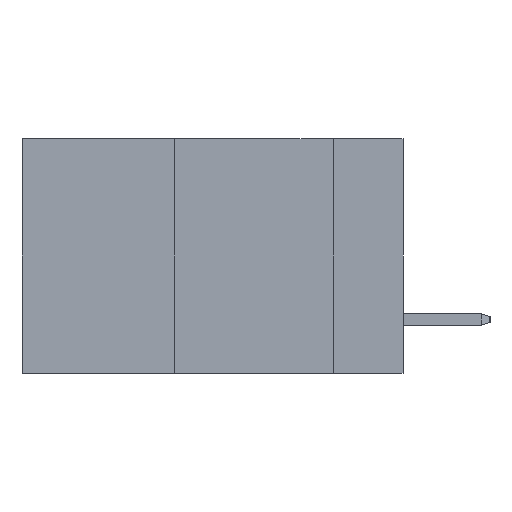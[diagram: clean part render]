
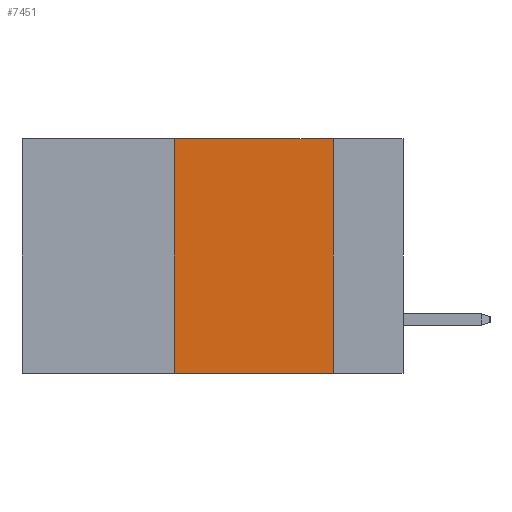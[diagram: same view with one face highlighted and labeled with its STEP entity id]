
A CAD part, left-side view. The second image highlights one B-rep face of the part: STEP entity #7451.
In plain terms, the highlighted planar face has unit normal (-1, 0, 0).
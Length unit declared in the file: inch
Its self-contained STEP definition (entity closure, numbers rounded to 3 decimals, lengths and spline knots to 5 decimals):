
#170 = DIRECTION ( 'NONE',  ( 0., -1., 0. ) ) ;
#464 = EDGE_CURVE ( 'NONE', #6376, #3207, #1297, .T. ) ;
#1163 = DIRECTION ( 'NONE',  ( 1., 0., 0. ) ) ;
#1297 = LINE ( 'NONE', #16096, #6875 ) ;
#2264 = CARTESIAN_POINT ( 'NONE',  ( 0., 0.36, 0. ) ) ;
#2473 = CARTESIAN_POINT ( 'NONE',  ( 0., 0.36, 0. ) ) ;
#2484 = PLANE ( 'NONE',  #2723 ) ;
#2723 = AXIS2_PLACEMENT_3D ( 'NONE', #7893, #1163, #16060 ) ;
#3059 = LINE ( 'NONE', #8479, #6296 ) ;
#3207 = VERTEX_POINT ( 'NONE', #8683 ) ;
#3241 = LINE ( 'NONE', #16770, #14973 ) ;
#3449 = ORIENTED_EDGE ( 'NONE', *, *, #464, .F. ) ;
#3927 = CARTESIAN_POINT ( 'NONE',  ( 0., 0.11, 0. ) ) ;
#6296 = VECTOR ( 'NONE', #12302, 39.37008 ) ;
#6376 = VERTEX_POINT ( 'NONE', #3927 ) ;
#6842 = CARTESIAN_POINT ( 'NONE',  ( 0., 0.36, -0.37 ) ) ;
#6875 = VECTOR ( 'NONE', #17376, 39.37008 ) ;
#7451 = ADVANCED_FACE ( 'NONE', ( #14648 ), #2484, .F. ) ;
#7579 = LINE ( 'NONE', #2264, #11008 ) ;
#7796 = ORIENTED_EDGE ( 'NONE', *, *, #17082, .F. ) ;
#7893 = CARTESIAN_POINT ( 'NONE',  ( 0., 0.6, 0. ) ) ;
#8479 = CARTESIAN_POINT ( 'NONE',  ( 0., 0.6, 0. ) ) ;
#8683 = CARTESIAN_POINT ( 'NONE',  ( 0., 0.11, -0.37 ) ) ;
#9094 = ORIENTED_EDGE ( 'NONE', *, *, #9726, .T. ) ;
#9726 = EDGE_CURVE ( 'NONE', #10562, #3207, #3241, .T. ) ;
#9874 = EDGE_CURVE ( 'NONE', #10562, #12164, #7579, .T. ) ;
#10342 = DIRECTION ( 'NONE',  ( 0., 0., 1. ) ) ;
#10562 = VERTEX_POINT ( 'NONE', #6842 ) ;
#11008 = VECTOR ( 'NONE', #10342, 39.37008 ) ;
#12164 = VERTEX_POINT ( 'NONE', #2473 ) ;
#12302 = DIRECTION ( 'NONE',  ( 0., -1., 0. ) ) ;
#12348 = ORIENTED_EDGE ( 'NONE', *, *, #9874, .F. ) ;
#14312 = EDGE_LOOP ( 'NONE', ( #3449, #7796, #12348, #9094 ) ) ;
#14648 = FACE_OUTER_BOUND ( 'NONE', #14312, .T. ) ;
#14973 = VECTOR ( 'NONE', #170, 39.37008 ) ;
#16060 = DIRECTION ( 'NONE',  ( 0., 0., -1. ) ) ;
#16096 = CARTESIAN_POINT ( 'NONE',  ( 0., 0.11, 0. ) ) ;
#16770 = CARTESIAN_POINT ( 'NONE',  ( 0., 0.6, -0.37 ) ) ;
#17082 = EDGE_CURVE ( 'NONE', #12164, #6376, #3059, .T. ) ;
#17376 = DIRECTION ( 'NONE',  ( 0., 0., -1. ) ) ;
